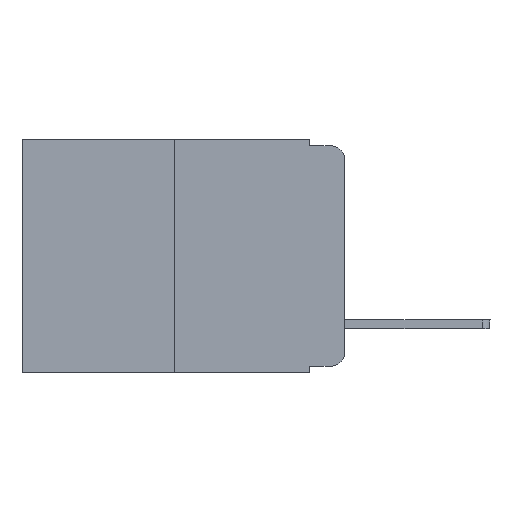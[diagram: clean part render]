
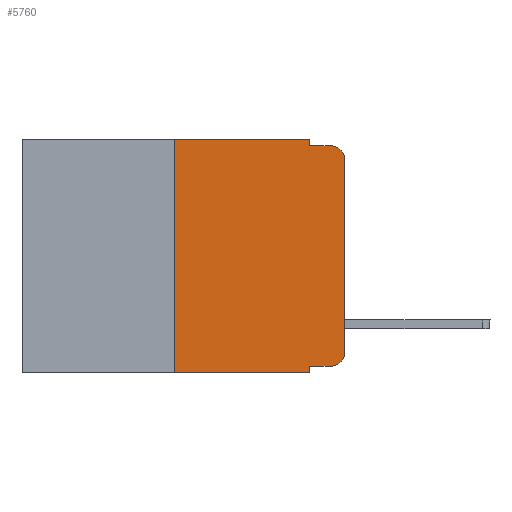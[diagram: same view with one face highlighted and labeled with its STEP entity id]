
A CAD part, left-side view. The second image highlights one B-rep face of the part: STEP entity #5760.
In plain terms, the highlighted planar face has unit normal (-1, 0, 0).
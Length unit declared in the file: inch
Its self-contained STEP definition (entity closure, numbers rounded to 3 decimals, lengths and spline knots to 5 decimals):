
#435 = CARTESIAN_POINT ( 'NONE',  ( 0., 0.473, 0. ) ) ;
#438 = EDGE_CURVE ( 'NONE', #11149, #2768, #2600, .T. ) ;
#526 = ORIENTED_EDGE ( 'NONE', *, *, #5381, .F. ) ;
#1446 = DIRECTION ( 'NONE',  ( 0., -1., 0. ) ) ;
#1843 = ORIENTED_EDGE ( 'NONE', *, *, #6966, .T. ) ;
#1984 = DIRECTION ( 'NONE',  ( 0., -1., 0. ) ) ;
#2387 = AXIS2_PLACEMENT_3D ( 'NONE', #5859, #11692, #13126 ) ;
#2510 = CARTESIAN_POINT ( 'NONE',  ( 0., 0.25, -0.343 ) ) ;
#2529 = VERTEX_POINT ( 'NONE', #4061 ) ;
#2582 = EDGE_LOOP ( 'NONE', ( #16996, #7041, #11507, #13180, #526, #12880, #3148, #14319, #1843, #6513 ) ) ;
#2600 = LINE ( 'NONE', #11429, #6575 ) ;
#2768 = VERTEX_POINT ( 'NONE', #10787 ) ;
#2845 = LINE ( 'NONE', #5293, #9784 ) ;
#2860 = CARTESIAN_POINT ( 'NONE',  ( 0., 0.473, -0.343 ) ) ;
#3148 = ORIENTED_EDGE ( 'NONE', *, *, #17185, .T. ) ;
#3394 = LINE ( 'NONE', #12152, #14358 ) ;
#4061 = CARTESIAN_POINT ( 'NONE',  ( 0., 0.051, -0.343 ) ) ;
#4760 = VECTOR ( 'NONE', #1446, 39.37008 ) ;
#4835 = CARTESIAN_POINT ( 'NONE',  ( 0., 0.051, 0. ) ) ;
#5293 = CARTESIAN_POINT ( 'NONE',  ( 0., 0.473, 0. ) ) ;
#5381 = EDGE_CURVE ( 'NONE', #9465, #10014, #2845, .T. ) ;
#5531 = LINE ( 'NONE', #11349, #14477 ) ;
#5760 = ADVANCED_FACE ( 'NONE', ( #13477 ), #16611, .F. ) ;
#5782 = EDGE_CURVE ( 'NONE', #14223, #11149, #5865, .T. ) ;
#5859 = CARTESIAN_POINT ( 'NONE',  ( 0., 0.02, -0.03 ) ) ;
#5865 = CIRCLE ( 'NONE', #8337, 0.02 ) ;
#5983 = VERTEX_POINT ( 'NONE', #13363 ) ;
#6036 = CARTESIAN_POINT ( 'NONE',  ( 0., 0.051, -0.333 ) ) ;
#6217 = DIRECTION ( 'NONE',  ( 0., 0., -1. ) ) ;
#6513 = ORIENTED_EDGE ( 'NONE', *, *, #5782, .T. ) ;
#6575 = VECTOR ( 'NONE', #7115, 39.37008 ) ;
#6966 = EDGE_CURVE ( 'NONE', #12180, #14223, #3394, .T. ) ;
#7041 = ORIENTED_EDGE ( 'NONE', *, *, #8975, .T. ) ;
#7115 = DIRECTION ( 'NONE',  ( 0., 0., 1. ) ) ;
#7339 = VERTEX_POINT ( 'NONE', #2510 ) ;
#7707 = CARTESIAN_POINT ( 'NONE',  ( 0., 0.051, -0.01 ) ) ;
#7767 = EDGE_CURVE ( 'NONE', #7339, #9465, #15604, .T. ) ;
#8337 = AXIS2_PLACEMENT_3D ( 'NONE', #16423, #9197, #14997 ) ;
#8629 = LINE ( 'NONE', #17464, #9531 ) ;
#8877 = DIRECTION ( 'NONE',  ( 0., -1., 0. ) ) ;
#8975 = EDGE_CURVE ( 'NONE', #2768, #5983, #15121, .T. ) ;
#9197 = DIRECTION ( 'NONE',  ( -1., 0., 0. ) ) ;
#9465 = VERTEX_POINT ( 'NONE', #17387 ) ;
#9531 = VECTOR ( 'NONE', #13179, 39.37008 ) ;
#9784 = VECTOR ( 'NONE', #14163, 39.37008 ) ;
#9793 = DIRECTION ( 'NONE',  ( 0., 0., 1. ) ) ;
#10014 = VERTEX_POINT ( 'NONE', #4835 ) ;
#10787 = CARTESIAN_POINT ( 'NONE',  ( 0., 0., -0.03 ) ) ;
#11149 = VERTEX_POINT ( 'NONE', #15936 ) ;
#11349 = CARTESIAN_POINT ( 'NONE',  ( 0., 0.051, 0. ) ) ;
#11429 = CARTESIAN_POINT ( 'NONE',  ( 0., 0., 0. ) ) ;
#11507 = ORIENTED_EDGE ( 'NONE', *, *, #13031, .F. ) ;
#11692 = DIRECTION ( 'NONE',  ( -1., 0., 0. ) ) ;
#11725 = CARTESIAN_POINT ( 'NONE',  ( 0., 0.02, -0.333 ) ) ;
#12152 = CARTESIAN_POINT ( 'NONE',  ( 0., 0.051, -0.333 ) ) ;
#12180 = VERTEX_POINT ( 'NONE', #6036 ) ;
#12880 = ORIENTED_EDGE ( 'NONE', *, *, #7767, .F. ) ;
#13031 = EDGE_CURVE ( 'NONE', #14859, #5983, #13431, .T. ) ;
#13126 = DIRECTION ( 'NONE',  ( 0., 0., -1. ) ) ;
#13179 = DIRECTION ( 'NONE',  ( 0., 0., -1. ) ) ;
#13180 = ORIENTED_EDGE ( 'NONE', *, *, #16534, .F. ) ;
#13363 = CARTESIAN_POINT ( 'NONE',  ( 0., 0.02, -0.01 ) ) ;
#13431 = LINE ( 'NONE', #7707, #13770 ) ;
#13477 = FACE_OUTER_BOUND ( 'NONE', #2582, .T. ) ;
#13591 = CARTESIAN_POINT ( 'NONE',  ( 0., 0.051, -0.01 ) ) ;
#13750 = EDGE_CURVE ( 'NONE', #12180, #2529, #8629, .T. ) ;
#13770 = VECTOR ( 'NONE', #8877, 39.37008 ) ;
#14163 = DIRECTION ( 'NONE',  ( 0., -1., 0. ) ) ;
#14223 = VERTEX_POINT ( 'NONE', #11725 ) ;
#14319 = ORIENTED_EDGE ( 'NONE', *, *, #13750, .F. ) ;
#14358 = VECTOR ( 'NONE', #1984, 39.37008 ) ;
#14424 = VECTOR ( 'NONE', #9793, 39.37008 ) ;
#14477 = VECTOR ( 'NONE', #18597, 39.37008 ) ;
#14859 = VERTEX_POINT ( 'NONE', #13591 ) ;
#14997 = DIRECTION ( 'NONE',  ( 0., 0., -1. ) ) ;
#15121 = CIRCLE ( 'NONE', #2387, 0.02 ) ;
#15604 = LINE ( 'NONE', #16844, #14424 ) ;
#15936 = CARTESIAN_POINT ( 'NONE',  ( 0., 0., -0.313 ) ) ;
#16260 = LINE ( 'NONE', #2860, #4760 ) ;
#16423 = CARTESIAN_POINT ( 'NONE',  ( 0., 0.02, -0.313 ) ) ;
#16534 = EDGE_CURVE ( 'NONE', #10014, #14859, #5531, .T. ) ;
#16611 = PLANE ( 'NONE',  #17737 ) ;
#16813 = DIRECTION ( 'NONE',  ( 1., 0., 0. ) ) ;
#16844 = CARTESIAN_POINT ( 'NONE',  ( 0., 0.25, 0. ) ) ;
#16996 = ORIENTED_EDGE ( 'NONE', *, *, #438, .T. ) ;
#17185 = EDGE_CURVE ( 'NONE', #7339, #2529, #16260, .T. ) ;
#17387 = CARTESIAN_POINT ( 'NONE',  ( 0., 0.25, 0. ) ) ;
#17464 = CARTESIAN_POINT ( 'NONE',  ( 0., 0.051, 0. ) ) ;
#17737 = AXIS2_PLACEMENT_3D ( 'NONE', #435, #16813, #6217 ) ;
#18597 = DIRECTION ( 'NONE',  ( 0., 0., -1. ) ) ;
